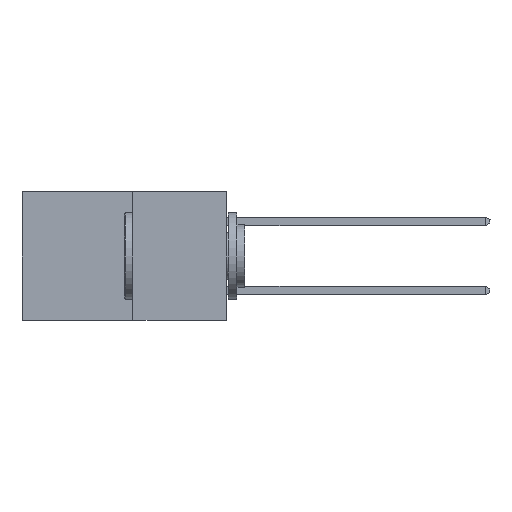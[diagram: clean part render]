
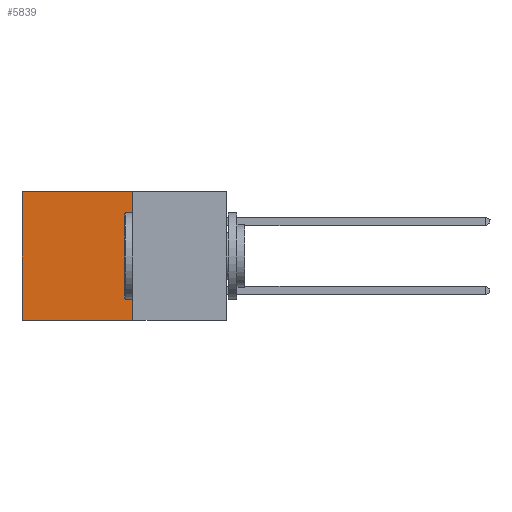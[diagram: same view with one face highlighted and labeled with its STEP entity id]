
A CAD part, left-side view. The second image highlights one B-rep face of the part: STEP entity #5839.
In plain terms, the highlighted planar face has unit normal (-1, 0, 0).
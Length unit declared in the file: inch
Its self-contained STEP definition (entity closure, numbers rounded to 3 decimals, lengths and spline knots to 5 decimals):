
#330 = DIRECTION ( 'NONE',  ( 0., 1., 0. ) ) ;
#2087 = LINE ( 'NONE', #9219, #7078 ) ;
#2392 = CARTESIAN_POINT ( 'NONE',  ( 0.277, 0.27, -0.37 ) ) ;
#3192 = CARTESIAN_POINT ( 'NONE',  ( 0.277, 0.27, -0.37 ) ) ;
#3475 = VERTEX_POINT ( 'NONE', #21740 ) ;
#4257 = EDGE_LOOP ( 'NONE', ( #15557, #11028, #19139, #10911 ) ) ;
#5392 = DIRECTION ( 'NONE',  ( 0., 0., -1. ) ) ;
#5414 = DIRECTION ( 'NONE',  ( 1., 0., 0. ) ) ;
#5465 = CARTESIAN_POINT ( 'NONE',  ( 0.277, 0.27, -0.37 ) ) ;
#5695 = PLANE ( 'NONE',  #8289 ) ;
#5839 = ADVANCED_FACE ( 'NONE', ( #15312 ), #5695, .F. ) ;
#6432 = VECTOR ( 'NONE', #11435, 39.37008 ) ;
#7078 = VECTOR ( 'NONE', #21933, 39.37008 ) ;
#7285 = VECTOR ( 'NONE', #15176, 39.37008 ) ;
#8289 = AXIS2_PLACEMENT_3D ( 'NONE', #5465, #5414, #5392 ) ;
#9219 = CARTESIAN_POINT ( 'NONE',  ( 0.277, 0.59, -0.37 ) ) ;
#10911 = ORIENTED_EDGE ( 'NONE', *, *, #17446, .T. ) ;
#11028 = ORIENTED_EDGE ( 'NONE', *, *, #18764, .F. ) ;
#11435 = DIRECTION ( 'NONE',  ( 0., 1., 0. ) ) ;
#11479 = CARTESIAN_POINT ( 'NONE',  ( 0.277, 0.27, 0. ) ) ;
#11504 = LINE ( 'NONE', #2392, #7285 ) ;
#11668 = EDGE_CURVE ( 'NONE', #17914, #18399, #11504, .T. ) ;
#12701 = VECTOR ( 'NONE', #330, 39.37008 ) ;
#14906 = CARTESIAN_POINT ( 'NONE',  ( 0.277, 0.59, -0.37 ) ) ;
#15176 = DIRECTION ( 'NONE',  ( 0., 0., -1. ) ) ;
#15312 = FACE_OUTER_BOUND ( 'NONE', #4257, .T. ) ;
#15557 = ORIENTED_EDGE ( 'NONE', *, *, #17266, .T. ) ;
#17266 = EDGE_CURVE ( 'NONE', #3475, #18740, #2087, .T. ) ;
#17446 = EDGE_CURVE ( 'NONE', #17914, #3475, #22413, .T. ) ;
#17914 = VERTEX_POINT ( 'NONE', #19928 ) ;
#18399 = VERTEX_POINT ( 'NONE', #3192 ) ;
#18740 = VERTEX_POINT ( 'NONE', #14906 ) ;
#18764 = EDGE_CURVE ( 'NONE', #18399, #18740, #20393, .T. ) ;
#19139 = ORIENTED_EDGE ( 'NONE', *, *, #11668, .F. ) ;
#19928 = CARTESIAN_POINT ( 'NONE',  ( 0.277, 0.27, 0. ) ) ;
#20393 = LINE ( 'NONE', #22348, #6432 ) ;
#21740 = CARTESIAN_POINT ( 'NONE',  ( 0.277, 0.59, 0. ) ) ;
#21933 = DIRECTION ( 'NONE',  ( 0., 0., -1. ) ) ;
#22348 = CARTESIAN_POINT ( 'NONE',  ( 0.277, 0.27, -0.37 ) ) ;
#22413 = LINE ( 'NONE', #11479, #12701 ) ;
